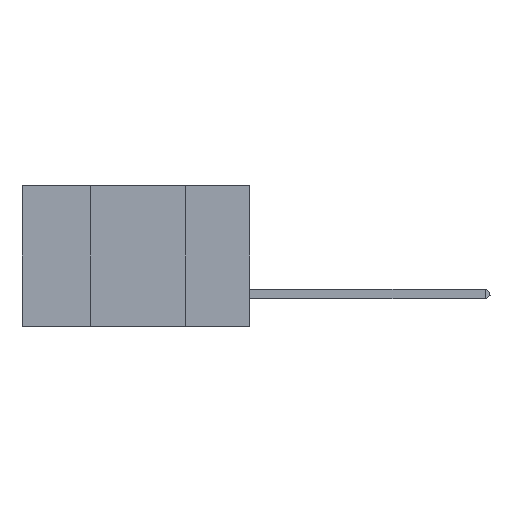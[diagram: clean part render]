
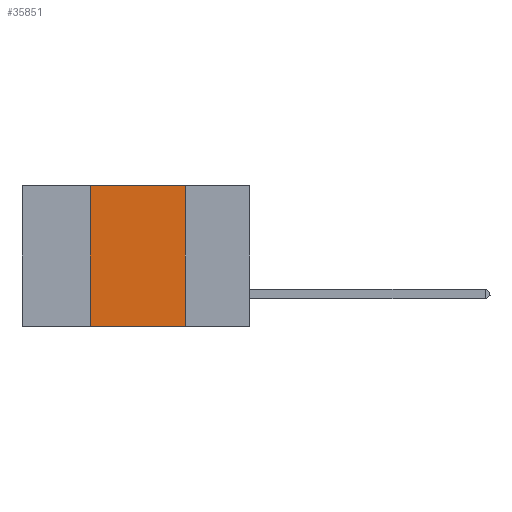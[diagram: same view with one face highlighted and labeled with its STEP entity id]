
A CAD part, left-side view. The second image highlights one B-rep face of the part: STEP entity #35851.
In plain terms, the highlighted planar face has unit normal (-1, 0, 0).
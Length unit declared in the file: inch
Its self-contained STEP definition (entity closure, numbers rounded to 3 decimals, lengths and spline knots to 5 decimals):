
#2610 = AXIS2_PLACEMENT_3D ( 'NONE', #24791, #24952, #35743 ) ;
#3274 = CARTESIAN_POINT ( 'NONE',  ( 0., 0.42, 0. ) ) ;
#3412 = LINE ( 'NONE', #18172, #37094 ) ;
#5347 = VERTEX_POINT ( 'NONE', #31434 ) ;
#9392 = ORIENTED_EDGE ( 'NONE', *, *, #23745, .F. ) ;
#10691 = VERTEX_POINT ( 'NONE', #24842 ) ;
#10777 = PLANE ( 'NONE',  #2610 ) ;
#10926 = EDGE_CURVE ( 'NONE', #5347, #41050, #19103, .T. ) ;
#12260 = DIRECTION ( 'NONE',  ( 0., 0., -1. ) ) ;
#12364 = VECTOR ( 'NONE', #31549, 39.37008 ) ;
#13521 = ORIENTED_EDGE ( 'NONE', *, *, #38676, .F. ) ;
#13566 = CARTESIAN_POINT ( 'NONE',  ( 0., 0.42, 0. ) ) ;
#18172 = CARTESIAN_POINT ( 'NONE',  ( 0., 0.6, -0.37 ) ) ;
#19103 = LINE ( 'NONE', #3274, #12364 ) ;
#21988 = DIRECTION ( 'NONE',  ( 0., -1., 0. ) ) ;
#23745 = EDGE_CURVE ( 'NONE', #41050, #41311, #24115, .T. ) ;
#23782 = ORIENTED_EDGE ( 'NONE', *, *, #10926, .F. ) ;
#24115 = LINE ( 'NONE', #28270, #33636 ) ;
#24783 = VECTOR ( 'NONE', #12260, 39.37008 ) ;
#24791 = CARTESIAN_POINT ( 'NONE',  ( 0., 0.6, 0. ) ) ;
#24842 = CARTESIAN_POINT ( 'NONE',  ( 0., 0.17, -0.37 ) ) ;
#24952 = DIRECTION ( 'NONE',  ( 1., 0., 0. ) ) ;
#25014 = DIRECTION ( 'NONE',  ( 0., -1., 0. ) ) ;
#25547 = ORIENTED_EDGE ( 'NONE', *, *, #35405, .T. ) ;
#28270 = CARTESIAN_POINT ( 'NONE',  ( 0., 0.6, 0. ) ) ;
#29706 = CARTESIAN_POINT ( 'NONE',  ( 0., 0.17, 0. ) ) ;
#31434 = CARTESIAN_POINT ( 'NONE',  ( 0., 0.42, -0.37 ) ) ;
#31477 = LINE ( 'NONE', #29706, #24783 ) ;
#31549 = DIRECTION ( 'NONE',  ( 0., 0., 1. ) ) ;
#32020 = FACE_OUTER_BOUND ( 'NONE', #34162, .T. ) ;
#33636 = VECTOR ( 'NONE', #25014, 39.37008 ) ;
#34162 = EDGE_LOOP ( 'NONE', ( #13521, #9392, #23782, #25547 ) ) ;
#35405 = EDGE_CURVE ( 'NONE', #5347, #10691, #3412, .T. ) ;
#35743 = DIRECTION ( 'NONE',  ( 0., 0., -1. ) ) ;
#35851 = ADVANCED_FACE ( 'NONE', ( #32020 ), #10777, .F. ) ;
#37094 = VECTOR ( 'NONE', #21988, 39.37008 ) ;
#38676 = EDGE_CURVE ( 'NONE', #41311, #10691, #31477, .T. ) ;
#41050 = VERTEX_POINT ( 'NONE', #13566 ) ;
#41311 = VERTEX_POINT ( 'NONE', #43600 ) ;
#43600 = CARTESIAN_POINT ( 'NONE',  ( 0., 0.17, 0. ) ) ;
